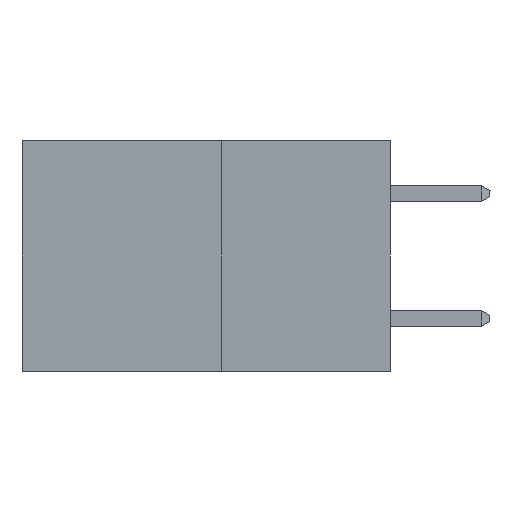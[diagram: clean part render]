
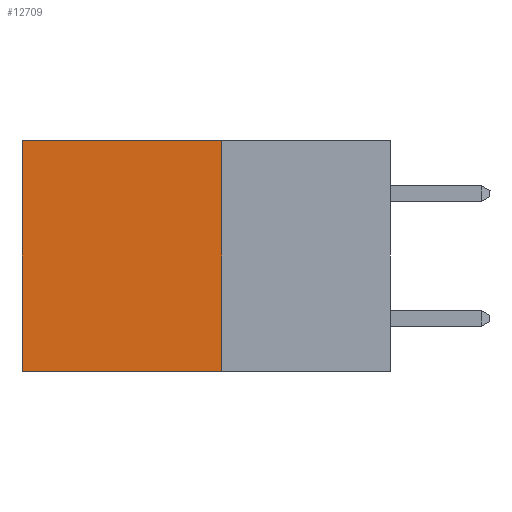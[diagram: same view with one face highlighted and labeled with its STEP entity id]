
A CAD part, left-side view. The second image highlights one B-rep face of the part: STEP entity #12709.
In plain terms, the highlighted planar face has unit normal (-1, 0, 0).
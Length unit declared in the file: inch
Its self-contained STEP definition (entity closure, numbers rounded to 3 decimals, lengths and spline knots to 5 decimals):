
#414 = LINE ( 'NONE', #3695, #11171 ) ;
#708 = EDGE_CURVE ( 'NONE', #12987, #8543, #12817, .T. ) ;
#906 = FACE_OUTER_BOUND ( 'NONE', #7917, .T. ) ;
#1516 = CARTESIAN_POINT ( 'NONE',  ( 0.277, 0.27, 0. ) ) ;
#2295 = VECTOR ( 'NONE', #8552, 39.37008 ) ;
#2438 = VECTOR ( 'NONE', #7663, 39.37008 ) ;
#2452 = ORIENTED_EDGE ( 'NONE', *, *, #8878, .T. ) ;
#2799 = ORIENTED_EDGE ( 'NONE', *, *, #708, .F. ) ;
#3358 = VECTOR ( 'NONE', #8558, 39.37008 ) ;
#3411 = ORIENTED_EDGE ( 'NONE', *, *, #9845, .T. ) ;
#3434 = CARTESIAN_POINT ( 'NONE',  ( 0.277, 0.27, -0.37 ) ) ;
#3695 = CARTESIAN_POINT ( 'NONE',  ( 0.277, 0.59, -0.37 ) ) ;
#3857 = EDGE_CURVE ( 'NONE', #8543, #4340, #8532, .T. ) ;
#4340 = VERTEX_POINT ( 'NONE', #7529 ) ;
#4865 = PLANE ( 'NONE',  #7058 ) ;
#5162 = CARTESIAN_POINT ( 'NONE',  ( 0.277, 0.27, -0.37 ) ) ;
#5713 = CARTESIAN_POINT ( 'NONE',  ( 0.277, 0.59, 0. ) ) ;
#5850 = DIRECTION ( 'NONE',  ( 0., 0., -1. ) ) ;
#7058 = AXIS2_PLACEMENT_3D ( 'NONE', #8667, #11566, #5850 ) ;
#7529 = CARTESIAN_POINT ( 'NONE',  ( 0.277, 0.59, -0.37 ) ) ;
#7663 = DIRECTION ( 'NONE',  ( 0., 0., -1. ) ) ;
#7843 = VERTEX_POINT ( 'NONE', #5713 ) ;
#7917 = EDGE_LOOP ( 'NONE', ( #3411, #11235, #2799, #2452 ) ) ;
#8500 = CARTESIAN_POINT ( 'NONE',  ( 0.277, 0.27, -0.37 ) ) ;
#8532 = LINE ( 'NONE', #8500, #3358 ) ;
#8543 = VERTEX_POINT ( 'NONE', #3434 ) ;
#8552 = DIRECTION ( 'NONE',  ( 0., 1., 0. ) ) ;
#8558 = DIRECTION ( 'NONE',  ( 0., 1., 0. ) ) ;
#8667 = CARTESIAN_POINT ( 'NONE',  ( 0.277, 0.27, -0.37 ) ) ;
#8878 = EDGE_CURVE ( 'NONE', #12987, #7843, #9561, .T. ) ;
#9561 = LINE ( 'NONE', #1516, #2295 ) ;
#9845 = EDGE_CURVE ( 'NONE', #7843, #4340, #414, .T. ) ;
#10440 = DIRECTION ( 'NONE',  ( 0., 0., -1. ) ) ;
#11053 = CARTESIAN_POINT ( 'NONE',  ( 0.277, 0.27, 0. ) ) ;
#11171 = VECTOR ( 'NONE', #10440, 39.37008 ) ;
#11235 = ORIENTED_EDGE ( 'NONE', *, *, #3857, .F. ) ;
#11566 = DIRECTION ( 'NONE',  ( 1., 0., 0. ) ) ;
#12709 = ADVANCED_FACE ( 'NONE', ( #906 ), #4865, .F. ) ;
#12817 = LINE ( 'NONE', #5162, #2438 ) ;
#12987 = VERTEX_POINT ( 'NONE', #11053 ) ;
